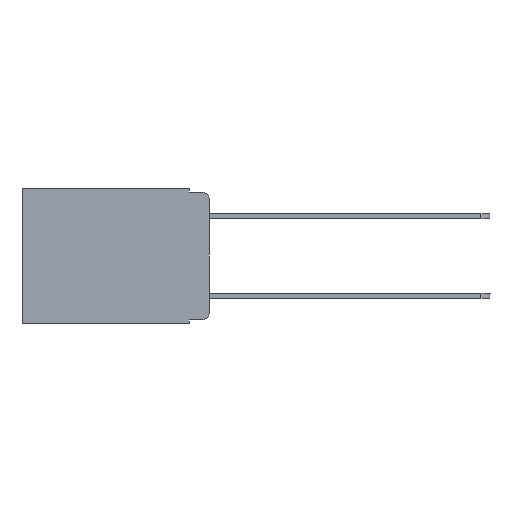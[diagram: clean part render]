
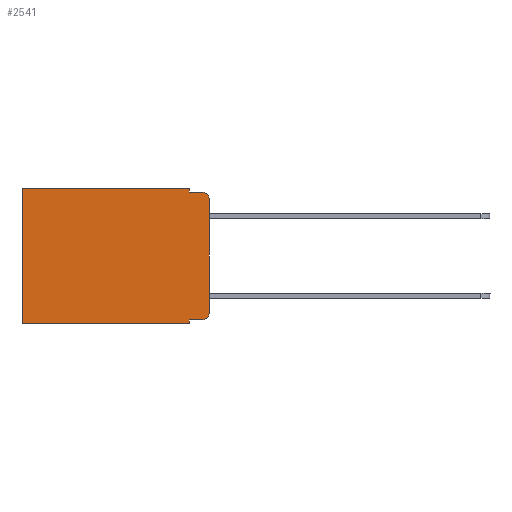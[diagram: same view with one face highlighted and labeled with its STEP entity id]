
A CAD part, left-side view. The second image highlights one B-rep face of the part: STEP entity #2541.
In plain terms, the highlighted planar face has unit normal (-1, 0, 0).
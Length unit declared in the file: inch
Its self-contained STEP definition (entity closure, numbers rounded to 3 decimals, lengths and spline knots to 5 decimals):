
#33 = EDGE_LOOP ( 'NONE', ( #6756, #7546, #5591, #8585, #4093, #6761, #9108, #8697, #7035, #7131 ) ) ;
#143 = CARTESIAN_POINT ( 'NONE',  ( 0.298, 0.051, 0. ) ) ;
#360 = CARTESIAN_POINT ( 'NONE',  ( 0.298, 0.02, -0.333 ) ) ;
#471 = DIRECTION ( 'NONE',  ( 0., 0., -1. ) ) ;
#607 = EDGE_CURVE ( 'NONE', #1648, #7732, #6976, .T. ) ;
#804 = LINE ( 'NONE', #7019, #8336 ) ;
#1595 = EDGE_CURVE ( 'NONE', #4693, #10201, #804, .T. ) ;
#1648 = VERTEX_POINT ( 'NONE', #8717 ) ;
#1860 = VECTOR ( 'NONE', #8002, 39.37008 ) ;
#1901 = VERTEX_POINT ( 'NONE', #8488 ) ;
#1926 = DIRECTION ( 'NONE',  ( 0., 0., -1. ) ) ;
#1990 = DIRECTION ( 'NONE',  ( -1., 0., 0. ) ) ;
#1993 = CARTESIAN_POINT ( 'NONE',  ( 0.298, 0.02, -0.03 ) ) ;
#2224 = VECTOR ( 'NONE', #4183, 39.37008 ) ;
#2272 = CARTESIAN_POINT ( 'NONE',  ( 0.298, 0., 0. ) ) ;
#2395 = CARTESIAN_POINT ( 'NONE',  ( 0.298, 0., 0. ) ) ;
#2427 = CARTESIAN_POINT ( 'NONE',  ( 0.298, 0.051, 0. ) ) ;
#2491 = LINE ( 'NONE', #5430, #2224 ) ;
#2541 = ADVANCED_FACE ( 'NONE', ( #3513 ), #7081, .F. ) ;
#2570 = VECTOR ( 'NONE', #3206, 39.37008 ) ;
#2737 = LINE ( 'NONE', #6495, #1860 ) ;
#2965 = VECTOR ( 'NONE', #9592, 39.37008 ) ;
#3001 = VERTEX_POINT ( 'NONE', #4417 ) ;
#3206 = DIRECTION ( 'NONE',  ( 0., 0., -1. ) ) ;
#3285 = VECTOR ( 'NONE', #4717, 39.37008 ) ;
#3513 = FACE_OUTER_BOUND ( 'NONE', #33, .T. ) ;
#3559 = DIRECTION ( 'NONE',  ( -1., 0., 0. ) ) ;
#3905 = LINE ( 'NONE', #2395, #3285 ) ;
#4093 = ORIENTED_EDGE ( 'NONE', *, *, #9467, .T. ) ;
#4183 = DIRECTION ( 'NONE',  ( 0., 1., 0. ) ) ;
#4272 = CARTESIAN_POINT ( 'NONE',  ( 0.298, 0.02, -0.313 ) ) ;
#4417 = CARTESIAN_POINT ( 'NONE',  ( 0.298, 0.051, -0.01 ) ) ;
#4491 = VERTEX_POINT ( 'NONE', #4885 ) ;
#4693 = VERTEX_POINT ( 'NONE', #8567 ) ;
#4717 = DIRECTION ( 'NONE',  ( 0., 1., 0. ) ) ;
#4885 = CARTESIAN_POINT ( 'NONE',  ( 0.298, 0.02, -0.01 ) ) ;
#4911 = EDGE_CURVE ( 'NONE', #1648, #7043, #2737, .T. ) ;
#4980 = DIRECTION ( 'NONE',  ( 0., 0., -1. ) ) ;
#5259 = CARTESIAN_POINT ( 'NONE',  ( 0.298, 0.473, -0.343 ) ) ;
#5430 = CARTESIAN_POINT ( 'NONE',  ( 0.298, 0., -0.343 ) ) ;
#5591 = ORIENTED_EDGE ( 'NONE', *, *, #5817, .F. ) ;
#5809 = EDGE_CURVE ( 'NONE', #7732, #8694, #2491, .T. ) ;
#5817 = EDGE_CURVE ( 'NONE', #3001, #4491, #8524, .T. ) ;
#5975 = EDGE_CURVE ( 'NONE', #1901, #8694, #6650, .T. ) ;
#6123 = CIRCLE ( 'NONE', #7891, 0.02 ) ;
#6193 = CARTESIAN_POINT ( 'NONE',  ( 0.298, 0.051, 0. ) ) ;
#6220 = DIRECTION ( 'NONE',  ( 0., 0., -1. ) ) ;
#6495 = CARTESIAN_POINT ( 'NONE',  ( 0.298, 0.051, -0.333 ) ) ;
#6512 = VECTOR ( 'NONE', #4980, 39.37008 ) ;
#6550 = CARTESIAN_POINT ( 'NONE',  ( 0.298, 0.473, 0. ) ) ;
#6635 = EDGE_CURVE ( 'NONE', #6782, #3001, #9156, .T. ) ;
#6650 = LINE ( 'NONE', #6550, #7638 ) ;
#6756 = ORIENTED_EDGE ( 'NONE', *, *, #1595, .F. ) ;
#6761 = ORIENTED_EDGE ( 'NONE', *, *, #5975, .T. ) ;
#6782 = VERTEX_POINT ( 'NONE', #6193 ) ;
#6976 = LINE ( 'NONE', #2427, #2570 ) ;
#7002 = CARTESIAN_POINT ( 'NONE',  ( 0.298, 0.051, -0.01 ) ) ;
#7019 = CARTESIAN_POINT ( 'NONE',  ( 0.298, 0., 0. ) ) ;
#7035 = ORIENTED_EDGE ( 'NONE', *, *, #4911, .T. ) ;
#7043 = VERTEX_POINT ( 'NONE', #360 ) ;
#7048 = DIRECTION ( 'NONE',  ( 1., 0., 0. ) ) ;
#7081 = PLANE ( 'NONE',  #10045 ) ;
#7131 = ORIENTED_EDGE ( 'NONE', *, *, #8552, .T. ) ;
#7546 = ORIENTED_EDGE ( 'NONE', *, *, #9861, .T. ) ;
#7638 = VECTOR ( 'NONE', #9054, 39.37008 ) ;
#7732 = VERTEX_POINT ( 'NONE', #8066 ) ;
#7786 = DIRECTION ( 'NONE',  ( 0., 0., -1. ) ) ;
#7891 = AXIS2_PLACEMENT_3D ( 'NONE', #4272, #1990, #1926 ) ;
#8002 = DIRECTION ( 'NONE',  ( 0., -1., 0. ) ) ;
#8066 = CARTESIAN_POINT ( 'NONE',  ( 0.298, 0.051, -0.343 ) ) ;
#8336 = VECTOR ( 'NONE', #7786, 39.37008 ) ;
#8488 = CARTESIAN_POINT ( 'NONE',  ( 0.298, 0.473, 0. ) ) ;
#8524 = LINE ( 'NONE', #7002, #2965 ) ;
#8552 = EDGE_CURVE ( 'NONE', #7043, #10201, #6123, .T. ) ;
#8567 = CARTESIAN_POINT ( 'NONE',  ( 0.298, 0., -0.03 ) ) ;
#8585 = ORIENTED_EDGE ( 'NONE', *, *, #6635, .F. ) ;
#8694 = VERTEX_POINT ( 'NONE', #5259 ) ;
#8697 = ORIENTED_EDGE ( 'NONE', *, *, #607, .F. ) ;
#8717 = CARTESIAN_POINT ( 'NONE',  ( 0.298, 0.051, -0.333 ) ) ;
#9054 = DIRECTION ( 'NONE',  ( 0., 0., -1. ) ) ;
#9108 = ORIENTED_EDGE ( 'NONE', *, *, #5809, .F. ) ;
#9156 = LINE ( 'NONE', #143, #6512 ) ;
#9467 = EDGE_CURVE ( 'NONE', #6782, #1901, #3905, .T. ) ;
#9592 = DIRECTION ( 'NONE',  ( 0., -1., 0. ) ) ;
#9600 = CARTESIAN_POINT ( 'NONE',  ( 0.298, 0., -0.313 ) ) ;
#9831 = CIRCLE ( 'NONE', #10231, 0.02 ) ;
#9861 = EDGE_CURVE ( 'NONE', #4693, #4491, #9831, .T. ) ;
#10045 = AXIS2_PLACEMENT_3D ( 'NONE', #2272, #7048, #6220 ) ;
#10201 = VERTEX_POINT ( 'NONE', #9600 ) ;
#10231 = AXIS2_PLACEMENT_3D ( 'NONE', #1993, #3559, #471 ) ;
